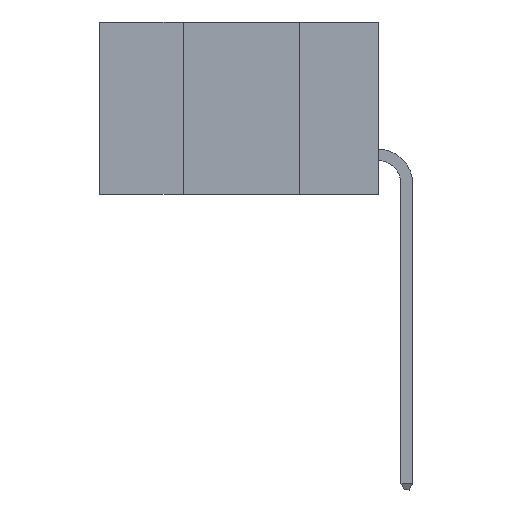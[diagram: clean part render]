
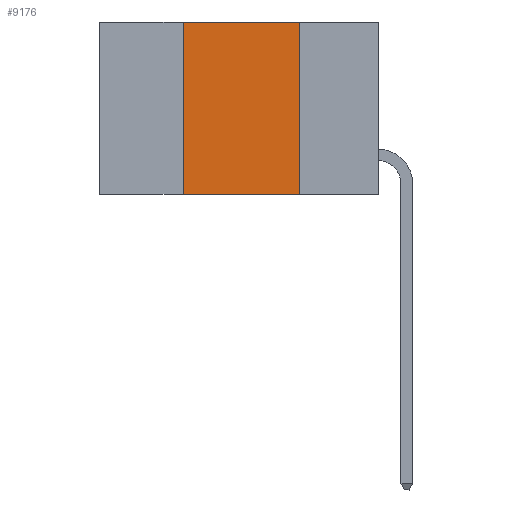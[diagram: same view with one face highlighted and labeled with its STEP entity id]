
A CAD part, left-side view. The second image highlights one B-rep face of the part: STEP entity #9176.
In plain terms, the highlighted planar face has unit normal (-1, 0, 0).
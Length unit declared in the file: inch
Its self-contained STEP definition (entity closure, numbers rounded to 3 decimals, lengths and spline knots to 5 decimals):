
#190 = VERTEX_POINT ( 'NONE', #7344 ) ;
#199 = AXIS2_PLACEMENT_3D ( 'NONE', #4494, #2395, #7506 ) ;
#790 = CARTESIAN_POINT ( 'NONE',  ( 0., 0.17, 0. ) ) ;
#1285 = ORIENTED_EDGE ( 'NONE', *, *, #1333, .F. ) ;
#1333 = EDGE_CURVE ( 'NONE', #8923, #11507, #9007, .T. ) ;
#1628 = CARTESIAN_POINT ( 'NONE',  ( 0., 0.17, 0. ) ) ;
#1689 = DIRECTION ( 'NONE',  ( 0., -1., 0. ) ) ;
#1816 = VECTOR ( 'NONE', #1689, 39.37008 ) ;
#2170 = VERTEX_POINT ( 'NONE', #790 ) ;
#2395 = DIRECTION ( 'NONE',  ( 1., 0., 0. ) ) ;
#4336 = VECTOR ( 'NONE', #5031, 39.37008 ) ;
#4494 = CARTESIAN_POINT ( 'NONE',  ( 0., 0.6, 0. ) ) ;
#4586 = CARTESIAN_POINT ( 'NONE',  ( 0., 0.42, 0. ) ) ;
#5031 = DIRECTION ( 'NONE',  ( 0., -1., 0. ) ) ;
#5452 = PLANE ( 'NONE',  #199 ) ;
#5476 = ORIENTED_EDGE ( 'NONE', *, *, #5664, .T. ) ;
#5658 = DIRECTION ( 'NONE',  ( 0., 0., -1. ) ) ;
#5664 = EDGE_CURVE ( 'NONE', #8923, #190, #11417, .T. ) ;
#5875 = VECTOR ( 'NONE', #5658, 39.37008 ) ;
#5930 = ORIENTED_EDGE ( 'NONE', *, *, #11958, .F. ) ;
#6291 = EDGE_LOOP ( 'NONE', ( #10554, #5930, #1285, #5476 ) ) ;
#6317 = VECTOR ( 'NONE', #7759, 39.37008 ) ;
#6687 = CARTESIAN_POINT ( 'NONE',  ( 0., 0.6, -0.37 ) ) ;
#6959 = EDGE_CURVE ( 'NONE', #2170, #190, #8556, .T. ) ;
#7344 = CARTESIAN_POINT ( 'NONE',  ( 0., 0.17, -0.37 ) ) ;
#7506 = DIRECTION ( 'NONE',  ( 0., 0., -1. ) ) ;
#7759 = DIRECTION ( 'NONE',  ( 0., 0., 1. ) ) ;
#8141 = CARTESIAN_POINT ( 'NONE',  ( 0., 0.42, -0.37 ) ) ;
#8556 = LINE ( 'NONE', #1628, #5875 ) ;
#8923 = VERTEX_POINT ( 'NONE', #8141 ) ;
#9007 = LINE ( 'NONE', #9727, #6317 ) ;
#9176 = ADVANCED_FACE ( 'NONE', ( #9270 ), #5452, .F. ) ;
#9270 = FACE_OUTER_BOUND ( 'NONE', #6291, .T. ) ;
#9727 = CARTESIAN_POINT ( 'NONE',  ( 0., 0.42, 0. ) ) ;
#10261 = CARTESIAN_POINT ( 'NONE',  ( 0., 0.6, 0. ) ) ;
#10554 = ORIENTED_EDGE ( 'NONE', *, *, #6959, .F. ) ;
#11417 = LINE ( 'NONE', #6687, #1816 ) ;
#11507 = VERTEX_POINT ( 'NONE', #4586 ) ;
#11911 = LINE ( 'NONE', #10261, #4336 ) ;
#11958 = EDGE_CURVE ( 'NONE', #11507, #2170, #11911, .T. ) ;
